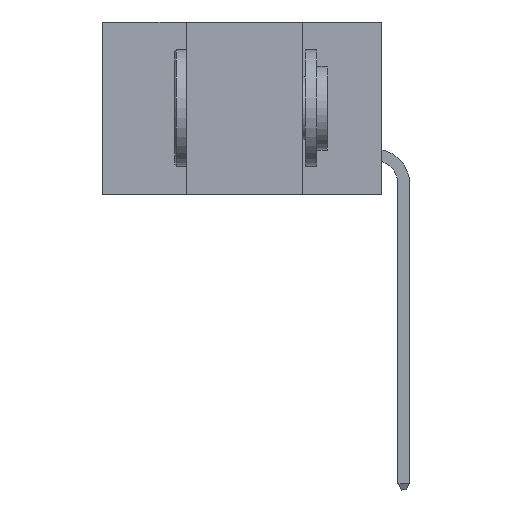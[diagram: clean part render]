
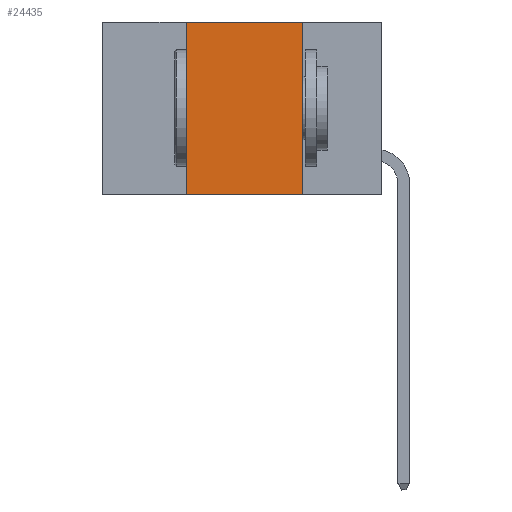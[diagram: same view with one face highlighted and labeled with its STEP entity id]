
A CAD part, left-side view. The second image highlights one B-rep face of the part: STEP entity #24435.
In plain terms, the highlighted planar face has unit normal (-1, 0, 0).
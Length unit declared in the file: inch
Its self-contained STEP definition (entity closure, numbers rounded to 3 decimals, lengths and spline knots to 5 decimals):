
#1743 = ORIENTED_EDGE ( 'NONE', *, *, #16469, .F. ) ;
#2023 = LINE ( 'NONE', #5781, #10203 ) ;
#2591 = CARTESIAN_POINT ( 'NONE',  ( 0., 0.42, 0. ) ) ;
#2870 = EDGE_CURVE ( 'NONE', #24027, #9557, #2023, .T. ) ;
#5781 = CARTESIAN_POINT ( 'NONE',  ( 0., 0.42, 0. ) ) ;
#6642 = DIRECTION ( 'NONE',  ( 0., -1., 0. ) ) ;
#7292 = DIRECTION ( 'NONE',  ( 1., 0., 0. ) ) ;
#9502 = DIRECTION ( 'NONE',  ( 0., 0., 1. ) ) ;
#9557 = VERTEX_POINT ( 'NONE', #2591 ) ;
#9776 = DIRECTION ( 'NONE',  ( 0., -1., 0. ) ) ;
#10203 = VECTOR ( 'NONE', #9502, 39.37008 ) ;
#10841 = CARTESIAN_POINT ( 'NONE',  ( 0., 0.17, 0. ) ) ;
#13476 = ORIENTED_EDGE ( 'NONE', *, *, #40718, .T. ) ;
#14202 = EDGE_LOOP ( 'NONE', ( #1743, #48639, #43528, #13476 ) ) ;
#15280 = VERTEX_POINT ( 'NONE', #47607 ) ;
#16469 = EDGE_CURVE ( 'NONE', #19170, #15280, #47167, .T. ) ;
#19170 = VERTEX_POINT ( 'NONE', #10841 ) ;
#19892 = EDGE_CURVE ( 'NONE', #9557, #19170, #38243, .T. ) ;
#21415 = CARTESIAN_POINT ( 'NONE',  ( 0., 0.6, 0. ) ) ;
#24027 = VERTEX_POINT ( 'NONE', #24054 ) ;
#24054 = CARTESIAN_POINT ( 'NONE',  ( 0., 0.42, -0.37 ) ) ;
#24435 = ADVANCED_FACE ( 'NONE', ( #41298 ), #29782, .F. ) ;
#27764 = VECTOR ( 'NONE', #9776, 39.37008 ) ;
#28254 = VECTOR ( 'NONE', #6642, 39.37008 ) ;
#29404 = AXIS2_PLACEMENT_3D ( 'NONE', #37352, #7292, #37824 ) ;
#29782 = PLANE ( 'NONE',  #29404 ) ;
#31236 = VECTOR ( 'NONE', #39644, 39.37008 ) ;
#36242 = CARTESIAN_POINT ( 'NONE',  ( 0., 0.6, -0.37 ) ) ;
#37352 = CARTESIAN_POINT ( 'NONE',  ( 0., 0.6, 0. ) ) ;
#37824 = DIRECTION ( 'NONE',  ( 0., 0., -1. ) ) ;
#38243 = LINE ( 'NONE', #21415, #28254 ) ;
#39644 = DIRECTION ( 'NONE',  ( 0., 0., -1. ) ) ;
#40125 = CARTESIAN_POINT ( 'NONE',  ( 0., 0.17, 0. ) ) ;
#40718 = EDGE_CURVE ( 'NONE', #24027, #15280, #46612, .T. ) ;
#41298 = FACE_OUTER_BOUND ( 'NONE', #14202, .T. ) ;
#43528 = ORIENTED_EDGE ( 'NONE', *, *, #2870, .F. ) ;
#46612 = LINE ( 'NONE', #36242, #27764 ) ;
#47167 = LINE ( 'NONE', #40125, #31236 ) ;
#47607 = CARTESIAN_POINT ( 'NONE',  ( 0., 0.17, -0.37 ) ) ;
#48639 = ORIENTED_EDGE ( 'NONE', *, *, #19892, .F. ) ;
